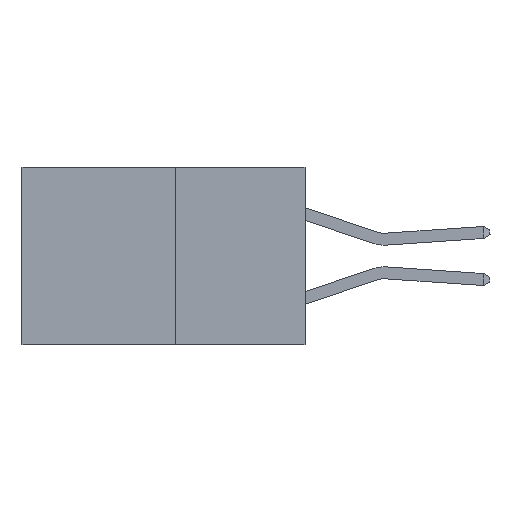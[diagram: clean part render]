
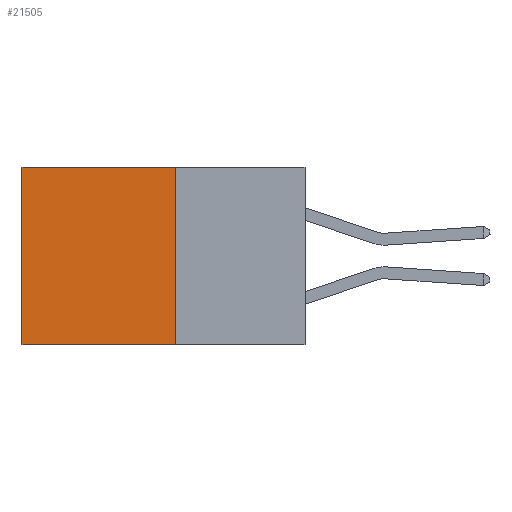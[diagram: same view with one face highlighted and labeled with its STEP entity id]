
A CAD part, left-side view. The second image highlights one B-rep face of the part: STEP entity #21505.
In plain terms, the highlighted planar face has unit normal (-1, 0, 0).
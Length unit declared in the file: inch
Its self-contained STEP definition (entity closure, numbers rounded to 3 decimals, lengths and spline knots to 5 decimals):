
#926 = LINE ( 'NONE', #13430, #10980 ) ;
#1257 = FACE_OUTER_BOUND ( 'NONE', #22633, .T. ) ;
#2874 = VERTEX_POINT ( 'NONE', #4453 ) ;
#3326 = VERTEX_POINT ( 'NONE', #10173 ) ;
#3717 = EDGE_CURVE ( 'NONE', #2874, #3326, #17089, .T. ) ;
#4453 = CARTESIAN_POINT ( 'NONE',  ( 0.277, 0.59, 0. ) ) ;
#4598 = EDGE_CURVE ( 'NONE', #5652, #2874, #13703, .T. ) ;
#4880 = DIRECTION ( 'NONE',  ( 0., 0., -1. ) ) ;
#5652 = VERTEX_POINT ( 'NONE', #6755 ) ;
#6685 = AXIS2_PLACEMENT_3D ( 'NONE', #14751, #16694, #4880 ) ;
#6755 = CARTESIAN_POINT ( 'NONE',  ( 0.277, 0.27, 0. ) ) ;
#8440 = VECTOR ( 'NONE', #9775, 39.37008 ) ;
#9775 = DIRECTION ( 'NONE',  ( 0., 1., 0. ) ) ;
#10173 = CARTESIAN_POINT ( 'NONE',  ( 0.277, 0.59, -0.37 ) ) ;
#10459 = EDGE_CURVE ( 'NONE', #5652, #12394, #15755, .T. ) ;
#10510 = VECTOR ( 'NONE', #10687, 39.37008 ) ;
#10687 = DIRECTION ( 'NONE',  ( 0., 0., -1. ) ) ;
#10980 = VECTOR ( 'NONE', #24980, 39.37008 ) ;
#12394 = VERTEX_POINT ( 'NONE', #20213 ) ;
#12499 = VECTOR ( 'NONE', #16890, 39.37008 ) ;
#12747 = PLANE ( 'NONE',  #6685 ) ;
#13430 = CARTESIAN_POINT ( 'NONE',  ( 0.277, 0.27, -0.37 ) ) ;
#13460 = ORIENTED_EDGE ( 'NONE', *, *, #10459, .F. ) ;
#13703 = LINE ( 'NONE', #17534, #8440 ) ;
#14751 = CARTESIAN_POINT ( 'NONE',  ( 0.277, 0.27, -0.37 ) ) ;
#15755 = LINE ( 'NONE', #16789, #10510 ) ;
#16524 = CARTESIAN_POINT ( 'NONE',  ( 0.277, 0.59, -0.37 ) ) ;
#16694 = DIRECTION ( 'NONE',  ( 1., 0., 0. ) ) ;
#16789 = CARTESIAN_POINT ( 'NONE',  ( 0.277, 0.27, -0.37 ) ) ;
#16823 = ORIENTED_EDGE ( 'NONE', *, *, #3717, .T. ) ;
#16890 = DIRECTION ( 'NONE',  ( 0., 0., -1. ) ) ;
#17089 = LINE ( 'NONE', #16524, #12499 ) ;
#17412 = ORIENTED_EDGE ( 'NONE', *, *, #21768, .F. ) ;
#17534 = CARTESIAN_POINT ( 'NONE',  ( 0.277, 0.27, 0. ) ) ;
#19781 = ORIENTED_EDGE ( 'NONE', *, *, #4598, .T. ) ;
#20213 = CARTESIAN_POINT ( 'NONE',  ( 0.277, 0.27, -0.37 ) ) ;
#21505 = ADVANCED_FACE ( 'NONE', ( #1257 ), #12747, .F. ) ;
#21768 = EDGE_CURVE ( 'NONE', #12394, #3326, #926, .T. ) ;
#22633 = EDGE_LOOP ( 'NONE', ( #16823, #17412, #13460, #19781 ) ) ;
#24980 = DIRECTION ( 'NONE',  ( 0., 1., 0. ) ) ;
